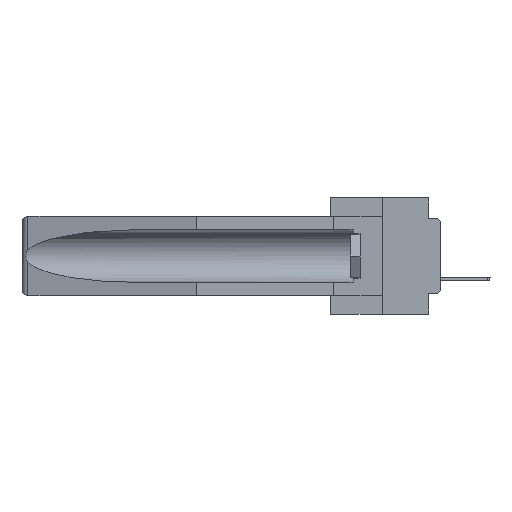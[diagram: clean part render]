
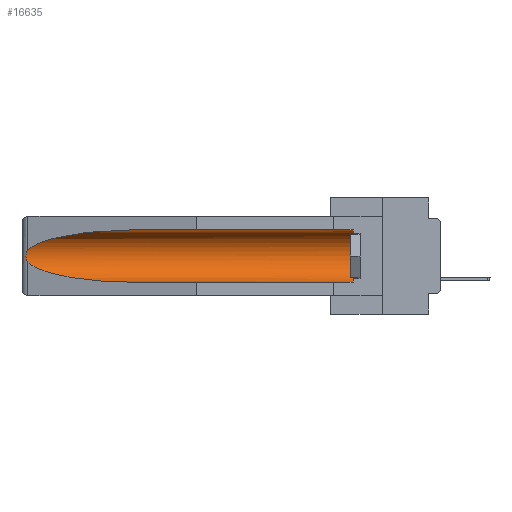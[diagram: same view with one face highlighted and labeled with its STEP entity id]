
A CAD part, left-side view. The second image highlights one B-rep face of the part: STEP entity #16635.
In plain terms, the highlighted cylindrical face has radius 2.857 mm (diameter 5.715 mm), a partial arc.
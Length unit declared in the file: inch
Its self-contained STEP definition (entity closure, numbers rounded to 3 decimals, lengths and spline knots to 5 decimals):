
#166 = DIRECTION ( 'NONE',  ( 0., 1., 0. ) ) ;
#1071 = CARTESIAN_POINT ( 'NONE',  ( 0.155, 1.07973, -0.059 ) ) ;
#1210 = DIRECTION ( 'NONE',  ( 0., 1., 0. ) ) ;
#2677 = FACE_OUTER_BOUND ( 'NONE', #14627, .T. ) ;
#3005 = CARTESIAN_POINT ( 'NONE',  ( 0.155, 1.07973, -0.059 ) ) ;
#3039 = AXIS2_PLACEMENT_3D ( 'NONE', #11612, #21231, #27964 ) ;
#4768 = ORIENTED_EDGE ( 'NONE', *, *, #25908, .T. ) ;
#5351 = CARTESIAN_POINT ( 'NONE',  ( 0.155, 0.126, -0.284 ) ) ;
#6082 = LINE ( 'NONE', #10793, #8875 ) ;
#6097 = CARTESIAN_POINT ( 'NONE',  ( 0.21114, 1.30732, -0.059 ) ) ;
#6578 =( BOUNDED_CURVE ( )  B_SPLINE_CURVE ( 3, ( #27254, #20181, #27398, #17989 ),
 .UNSPECIFIED., .F., .F. ) 
 B_SPLINE_CURVE_WITH_KNOTS ( ( 4, 4 ),
 ( 0.1948, 1.5708 ),
 .UNSPECIFIED. ) 
 CURVE ( )  GEOMETRIC_REPRESENTATION_ITEM ( )  RATIONAL_B_SPLINE_CURVE ( ( 1., 0.848, 0.848, 1. ) ) 
 REPRESENTATION_ITEM ( '' )  );
#7078 = VERTEX_POINT ( 'NONE', #28126 ) ;
#7383 = EDGE_CURVE ( 'NONE', #20198, #8293, #6082, .T. ) ;
#7460 = EDGE_CURVE ( 'NONE', #27534, #18016, #10640, .T. ) ;
#7778 = CARTESIAN_POINT ( 'NONE',  ( 0.2675, 1.53308, -0.17534 ) ) ;
#7852 = VECTOR ( 'NONE', #13482, 39.37008 ) ;
#8051 = CIRCLE ( 'NONE', #3039, 0.1125 ) ;
#8293 = VERTEX_POINT ( 'NONE', #27551 ) ;
#8403 = CARTESIAN_POINT ( 'NONE',  ( 0.2673, 1.53269, -0.17917 ) ) ;
#8875 = VECTOR ( 'NONE', #1210, 39.37008 ) ;
#10149 = CARTESIAN_POINT ( 'NONE',  ( 0.2675, 1.53308, -0.16763 ) ) ;
#10640 = LINE ( 'NONE', #20239, #7852 ) ;
#10793 = CARTESIAN_POINT ( 'NONE',  ( 0.155, -0.30754, -0.284 ) ) ;
#11612 = CARTESIAN_POINT ( 'NONE',  ( 0.155, 0.126, -0.1715 ) ) ;
#11656 = ORIENTED_EDGE ( 'NONE', *, *, #7460, .T. ) ;
#11889 = ORIENTED_EDGE ( 'NONE', *, *, #26720, .T. ) ;
#12827 = CARTESIAN_POINT ( 'NONE',  ( 0.2673, 1.5327, -0.16383 ) ) ;
#12864 = CARTESIAN_POINT ( 'NONE',  ( 0.26537, 1.52718, -0.14972 ) ) ;
#12877 = EDGE_CURVE ( 'NONE', #20198, #27534, #8051, .T. ) ;
#13482 = DIRECTION ( 'NONE',  ( 0., 1., 0. ) ) ;
#14627 = EDGE_LOOP ( 'NONE', ( #4768, #23465, #11889, #19565, #15714, #11656 ) ) ;
#14940 = CARTESIAN_POINT ( 'NONE',  ( 0.26537, 1.52718, -0.19328 ) ) ;
#15178 = CARTESIAN_POINT ( 'NONE',  ( 0.26597, 1.5296, -0.19026 ) ) ;
#15714 = ORIENTED_EDGE ( 'NONE', *, *, #12877, .T. ) ;
#16635 = ADVANCED_FACE ( 'NONE', ( #2677 ), #23923, .F. ) ;
#17855 = CARTESIAN_POINT ( 'NONE',  ( 0.26537, 1.52718, -0.19328 ) ) ;
#17989 = CARTESIAN_POINT ( 'NONE',  ( 0.155, 1.07973, -0.284 ) ) ;
#18016 = VERTEX_POINT ( 'NONE', #3005 ) ;
#18249 = B_SPLINE_CURVE_WITH_KNOTS ( 'NONE', 3,
 ( #29946, #25089, #22583, #12827, #10149, #7778, #8403, #22279, #15178, #17855 ),
 .UNSPECIFIED., .F., .F.,
 ( 4, 2, 2, 2, 4 ),
 ( 0., 0.00029, 0.00058, 0.00087, 0.00117 ),
 .UNSPECIFIED. ) ;
#18432 =( BOUNDED_CURVE ( )  B_SPLINE_CURVE ( 3, ( #1071, #6097, #20255, #12864 ),
 .UNSPECIFIED., .F., .F. ) 
 B_SPLINE_CURVE_WITH_KNOTS ( ( 4, 4 ),
 ( 4.71239, 6.08839 ),
 .UNSPECIFIED. ) 
 CURVE ( )  GEOMETRIC_REPRESENTATION_ITEM ( )  RATIONAL_B_SPLINE_CURVE ( ( 1., 0.848, 0.848, 1. ) ) 
 REPRESENTATION_ITEM ( '' )  );
#19565 = ORIENTED_EDGE ( 'NONE', *, *, #7383, .F. ) ;
#20181 = CARTESIAN_POINT ( 'NONE',  ( 0.25451, 1.48313, -0.24835 ) ) ;
#20198 = VERTEX_POINT ( 'NONE', #5351 ) ;
#20239 = CARTESIAN_POINT ( 'NONE',  ( 0.155, -0.30754, -0.059 ) ) ;
#20255 = CARTESIAN_POINT ( 'NONE',  ( 0.25451, 1.48313, -0.09465 ) ) ;
#21231 = DIRECTION ( 'NONE',  ( 0., -1., 0. ) ) ;
#21582 = CARTESIAN_POINT ( 'NONE',  ( 0.155, 0.126, -0.059 ) ) ;
#21884 = DIRECTION ( 'NONE',  ( 0., 0., 1. ) ) ;
#22279 = CARTESIAN_POINT ( 'NONE',  ( 0.26655, 1.53094, -0.18657 ) ) ;
#22583 = CARTESIAN_POINT ( 'NONE',  ( 0.26654, 1.53092, -0.15636 ) ) ;
#23465 = ORIENTED_EDGE ( 'NONE', *, *, #29838, .T. ) ;
#23923 = CYLINDRICAL_SURFACE ( 'NONE', #30259, 0.1125 ) ;
#23940 = VERTEX_POINT ( 'NONE', #14940 ) ;
#25089 = CARTESIAN_POINT ( 'NONE',  ( 0.26597, 1.52961, -0.15275 ) ) ;
#25908 = EDGE_CURVE ( 'NONE', #18016, #7078, #18432, .T. ) ;
#26720 = EDGE_CURVE ( 'NONE', #23940, #8293, #6578, .T. ) ;
#27254 = CARTESIAN_POINT ( 'NONE',  ( 0.26537, 1.52718, -0.19328 ) ) ;
#27398 = CARTESIAN_POINT ( 'NONE',  ( 0.21114, 1.30732, -0.284 ) ) ;
#27534 = VERTEX_POINT ( 'NONE', #21582 ) ;
#27551 = CARTESIAN_POINT ( 'NONE',  ( 0.155, 1.07973, -0.284 ) ) ;
#27964 = DIRECTION ( 'NONE',  ( 0., 0., 1. ) ) ;
#28126 = CARTESIAN_POINT ( 'NONE',  ( 0.26537, 1.52718, -0.14972 ) ) ;
#28479 = CARTESIAN_POINT ( 'NONE',  ( 0.155, -0.30754, -0.1715 ) ) ;
#29838 = EDGE_CURVE ( 'NONE', #7078, #23940, #18249, .T. ) ;
#29946 = CARTESIAN_POINT ( 'NONE',  ( 0.26537, 1.52718, -0.14972 ) ) ;
#30259 = AXIS2_PLACEMENT_3D ( 'NONE', #28479, #166, #21884 ) ;
